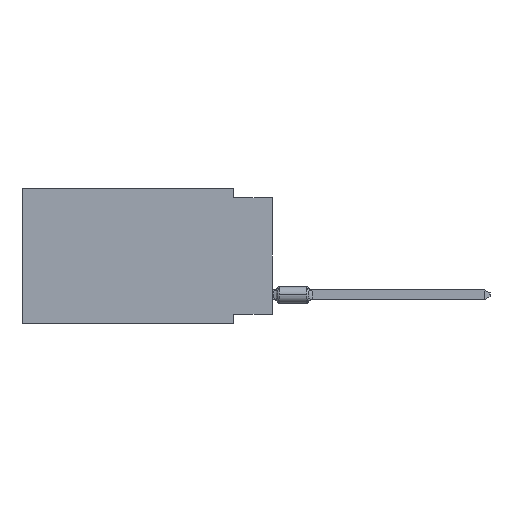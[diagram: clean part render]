
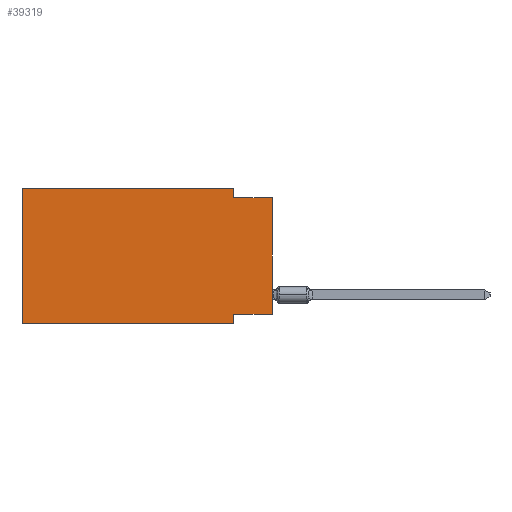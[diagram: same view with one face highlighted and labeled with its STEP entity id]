
A CAD part, left-side view. The second image highlights one B-rep face of the part: STEP entity #39319.
In plain terms, the highlighted planar face has unit normal (-1, 0, 0).
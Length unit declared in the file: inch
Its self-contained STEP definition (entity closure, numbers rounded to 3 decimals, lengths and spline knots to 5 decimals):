
#373 = FACE_OUTER_BOUND ( 'NONE', #14870, .T. ) ;
#6182 = CARTESIAN_POINT ( 'NONE',  ( 0., 0., -0.025 ) ) ;
#6389 = ORIENTED_EDGE ( 'NONE', *, *, #17964, .F. ) ;
#6676 = VECTOR ( 'NONE', #25314, 39.37008 ) ;
#6974 = EDGE_CURVE ( 'NONE', #7408, #46573, #11272, .T. ) ;
#7042 = VERTEX_POINT ( 'NONE', #22294 ) ;
#7408 = VERTEX_POINT ( 'NONE', #8077 ) ;
#7905 = DIRECTION ( 'NONE',  ( 0., 1., 0. ) ) ;
#8077 = CARTESIAN_POINT ( 'NONE',  ( 0., 0., -0.325 ) ) ;
#10098 = LINE ( 'NONE', #23774, #19448 ) ;
#10154 = DIRECTION ( 'NONE',  ( 0., 0., 1. ) ) ;
#10161 = CARTESIAN_POINT ( 'NONE',  ( 0., 0.1, 0. ) ) ;
#10223 = VECTOR ( 'NONE', #7905, 39.37008 ) ;
#10693 = LINE ( 'NONE', #35859, #6676 ) ;
#11170 = CARTESIAN_POINT ( 'NONE',  ( 0., 0.1, -0.325 ) ) ;
#11272 = LINE ( 'NONE', #23015, #10223 ) ;
#11465 = PLANE ( 'NONE',  #41434 ) ;
#11985 = EDGE_CURVE ( 'NONE', #7042, #30698, #10693, .T. ) ;
#12172 = DIRECTION ( 'NONE',  ( 1., 0., 0. ) ) ;
#12941 = EDGE_CURVE ( 'NONE', #7408, #17109, #43735, .T. ) ;
#13347 = VECTOR ( 'NONE', #31753, 39.37008 ) ;
#14870 = EDGE_LOOP ( 'NONE', ( #20739, #18492, #22909, #29971, #6389, #32159, #44905, #20218 ) ) ;
#17109 = VERTEX_POINT ( 'NONE', #6182 ) ;
#17579 = LINE ( 'NONE', #43478, #26826 ) ;
#17964 = EDGE_CURVE ( 'NONE', #23384, #7042, #17579, .T. ) ;
#18492 = ORIENTED_EDGE ( 'NONE', *, *, #33968, .F. ) ;
#19448 = VECTOR ( 'NONE', #38417, 39.37008 ) ;
#20218 = ORIENTED_EDGE ( 'NONE', *, *, #6974, .F. ) ;
#20720 = DIRECTION ( 'NONE',  ( 0., -1., 0. ) ) ;
#20739 = ORIENTED_EDGE ( 'NONE', *, *, #12941, .T. ) ;
#21706 = CARTESIAN_POINT ( 'NONE',  ( 0., 0.1, -0.35 ) ) ;
#22103 = EDGE_CURVE ( 'NONE', #30698, #32440, #42561, .T. ) ;
#22294 = CARTESIAN_POINT ( 'NONE',  ( 0., 0.645, 0. ) ) ;
#22909 = ORIENTED_EDGE ( 'NONE', *, *, #22103, .F. ) ;
#23015 = CARTESIAN_POINT ( 'NONE',  ( 0., 0., -0.325 ) ) ;
#23024 = EDGE_CURVE ( 'NONE', #46573, #30652, #25061, .T. ) ;
#23384 = VERTEX_POINT ( 'NONE', #43272 ) ;
#23774 = CARTESIAN_POINT ( 'NONE',  ( 0., 0., -0.025 ) ) ;
#25061 = LINE ( 'NONE', #21706, #40934 ) ;
#25244 = CARTESIAN_POINT ( 'NONE',  ( 0., 0., 0. ) ) ;
#25314 = DIRECTION ( 'NONE',  ( 0., -1., 0. ) ) ;
#25923 = CARTESIAN_POINT ( 'NONE',  ( 0., 0.1, 0. ) ) ;
#26826 = VECTOR ( 'NONE', #10154, 39.37008 ) ;
#29971 = ORIENTED_EDGE ( 'NONE', *, *, #11985, .F. ) ;
#30149 = DIRECTION ( 'NONE',  ( 0., 0., -1. ) ) ;
#30652 = VERTEX_POINT ( 'NONE', #32678 ) ;
#30698 = VERTEX_POINT ( 'NONE', #25923 ) ;
#31713 = EDGE_CURVE ( 'NONE', #23384, #30652, #38949, .T. ) ;
#31753 = DIRECTION ( 'NONE',  ( 0., 0., -1. ) ) ;
#32159 = ORIENTED_EDGE ( 'NONE', *, *, #31713, .T. ) ;
#32440 = VERTEX_POINT ( 'NONE', #41239 ) ;
#32678 = CARTESIAN_POINT ( 'NONE',  ( 0., 0.1, -0.35 ) ) ;
#33968 = EDGE_CURVE ( 'NONE', #32440, #17109, #10098, .T. ) ;
#35798 = CARTESIAN_POINT ( 'NONE',  ( 0., 0.645, -0.35 ) ) ;
#35859 = CARTESIAN_POINT ( 'NONE',  ( 0., 0.645, 0. ) ) ;
#38417 = DIRECTION ( 'NONE',  ( 0., -1., 0. ) ) ;
#38949 = LINE ( 'NONE', #35798, #40862 ) ;
#39319 = ADVANCED_FACE ( 'NONE', ( #373 ), #11465, .F. ) ;
#40862 = VECTOR ( 'NONE', #20720, 39.37008 ) ;
#40934 = VECTOR ( 'NONE', #46695, 39.37008 ) ;
#41239 = CARTESIAN_POINT ( 'NONE',  ( 0., 0.1, -0.025 ) ) ;
#41434 = AXIS2_PLACEMENT_3D ( 'NONE', #44803, #12172, #30149 ) ;
#42561 = LINE ( 'NONE', #10161, #13347 ) ;
#43262 = DIRECTION ( 'NONE',  ( 0., 0., 1. ) ) ;
#43272 = CARTESIAN_POINT ( 'NONE',  ( 0., 0.645, -0.35 ) ) ;
#43478 = CARTESIAN_POINT ( 'NONE',  ( 0., 0.645, 0. ) ) ;
#43735 = LINE ( 'NONE', #25244, #44294 ) ;
#44294 = VECTOR ( 'NONE', #43262, 39.37008 ) ;
#44803 = CARTESIAN_POINT ( 'NONE',  ( 0., 0.645, 0. ) ) ;
#44905 = ORIENTED_EDGE ( 'NONE', *, *, #23024, .F. ) ;
#46573 = VERTEX_POINT ( 'NONE', #11170 ) ;
#46695 = DIRECTION ( 'NONE',  ( 0., 0., -1. ) ) ;
